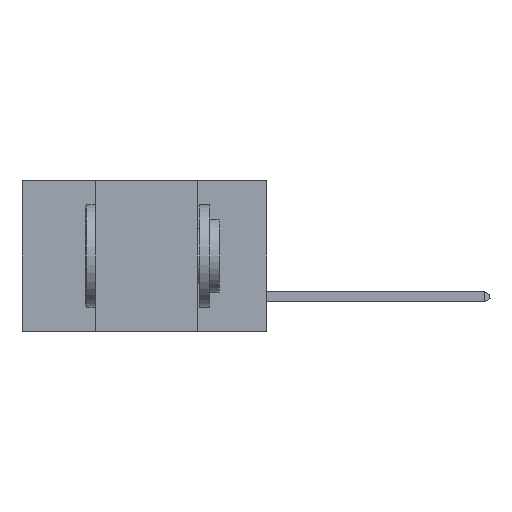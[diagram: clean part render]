
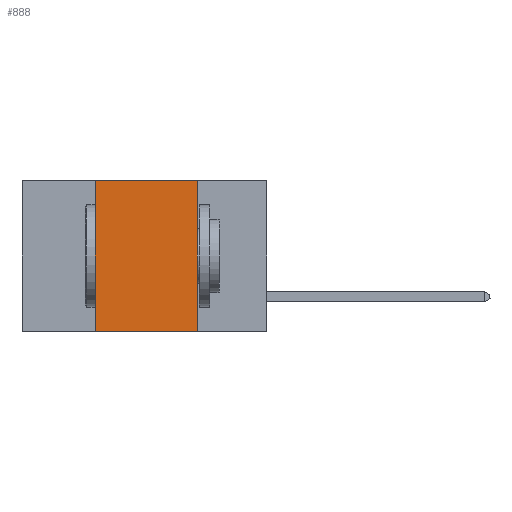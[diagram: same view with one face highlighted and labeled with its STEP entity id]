
A CAD part, left-side view. The second image highlights one B-rep face of the part: STEP entity #888.
In plain terms, the highlighted planar face has unit normal (-1, 0, 0).
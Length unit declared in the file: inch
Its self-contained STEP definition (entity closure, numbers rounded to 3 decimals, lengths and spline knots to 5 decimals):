
#212 = VECTOR ( 'NONE', #10363, 39.37008 ) ;
#542 = ORIENTED_EDGE ( 'NONE', *, *, #17007, .F. ) ;
#883 = FACE_OUTER_BOUND ( 'NONE', #6218, .T. ) ;
#888 = ADVANCED_FACE ( 'NONE', ( #883 ), #5798, .F. ) ;
#5053 = VERTEX_POINT ( 'NONE', #5891 ) ;
#5538 = DIRECTION ( 'NONE',  ( 0., 0., -1. ) ) ;
#5598 = DIRECTION ( 'NONE',  ( 1., 0., 0. ) ) ;
#5674 = CARTESIAN_POINT ( 'NONE',  ( 0., 0.6, 0. ) ) ;
#5798 = PLANE ( 'NONE',  #10045 ) ;
#5891 = CARTESIAN_POINT ( 'NONE',  ( 0., 0.17, 0. ) ) ;
#6040 = VECTOR ( 'NONE', #16282, 39.37008 ) ;
#6218 = EDGE_LOOP ( 'NONE', ( #542, #19715, #6502, #7053 ) ) ;
#6485 = VERTEX_POINT ( 'NONE', #17211 ) ;
#6502 = ORIENTED_EDGE ( 'NONE', *, *, #12451, .F. ) ;
#6830 = CARTESIAN_POINT ( 'NONE',  ( 0., 0.6, -0.37 ) ) ;
#7053 = ORIENTED_EDGE ( 'NONE', *, *, #18603, .T. ) ;
#7351 = VECTOR ( 'NONE', #13590, 39.37008 ) ;
#7917 = LINE ( 'NONE', #10115, #7351 ) ;
#8383 = VECTOR ( 'NONE', #10075, 39.37008 ) ;
#9620 = VERTEX_POINT ( 'NONE', #16171 ) ;
#10045 = AXIS2_PLACEMENT_3D ( 'NONE', #5674, #5598, #5538 ) ;
#10075 = DIRECTION ( 'NONE',  ( 0., 0., -1. ) ) ;
#10115 = CARTESIAN_POINT ( 'NONE',  ( 0., 0.6, 0. ) ) ;
#10363 = DIRECTION ( 'NONE',  ( 0., -1., 0. ) ) ;
#12242 = CARTESIAN_POINT ( 'NONE',  ( 0., 0.42, -0.37 ) ) ;
#12451 = EDGE_CURVE ( 'NONE', #15939, #6485, #19315, .T. ) ;
#13590 = DIRECTION ( 'NONE',  ( 0., -1., 0. ) ) ;
#14592 = CARTESIAN_POINT ( 'NONE',  ( 0., 0.42, 0. ) ) ;
#14851 = LINE ( 'NONE', #6830, #212 ) ;
#15939 = VERTEX_POINT ( 'NONE', #12242 ) ;
#16171 = CARTESIAN_POINT ( 'NONE',  ( 0., 0.17, -0.37 ) ) ;
#16282 = DIRECTION ( 'NONE',  ( 0., 0., 1. ) ) ;
#16965 = LINE ( 'NONE', #21967, #8383 ) ;
#17007 = EDGE_CURVE ( 'NONE', #5053, #9620, #16965, .T. ) ;
#17181 = EDGE_CURVE ( 'NONE', #6485, #5053, #7917, .T. ) ;
#17211 = CARTESIAN_POINT ( 'NONE',  ( 0., 0.42, 0. ) ) ;
#18603 = EDGE_CURVE ( 'NONE', #15939, #9620, #14851, .T. ) ;
#19315 = LINE ( 'NONE', #14592, #6040 ) ;
#19715 = ORIENTED_EDGE ( 'NONE', *, *, #17181, .F. ) ;
#21967 = CARTESIAN_POINT ( 'NONE',  ( 0., 0.17, 0. ) ) ;
